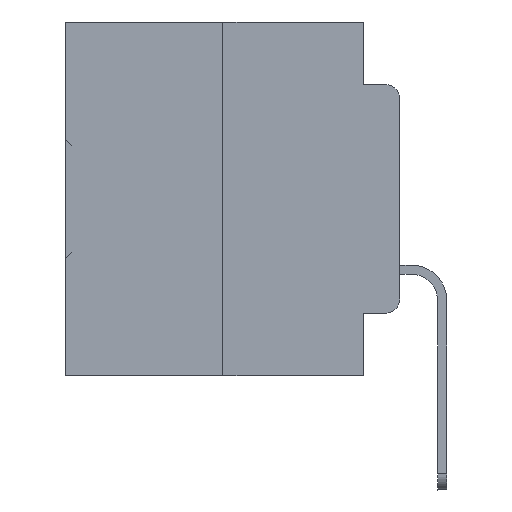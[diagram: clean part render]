
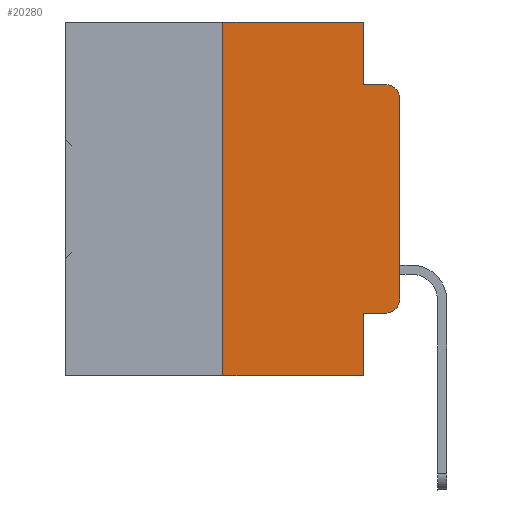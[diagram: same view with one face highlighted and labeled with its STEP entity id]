
A CAD part, left-side view. The second image highlights one B-rep face of the part: STEP entity #20280.
In plain terms, the highlighted planar face has unit normal (-1, 0, 0).
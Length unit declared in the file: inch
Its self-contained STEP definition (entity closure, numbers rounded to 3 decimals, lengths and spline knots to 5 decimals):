
#618 = AXIS2_PLACEMENT_3D ( 'NONE', #20040, #6520, #17661 ) ;
#851 = CARTESIAN_POINT ( 'NONE',  ( 0., 0.02, -0.4115 ) ) ;
#1379 = DIRECTION ( 'NONE',  ( 0., 0., -1. ) ) ;
#1526 = CARTESIAN_POINT ( 'NONE',  ( 0., 0.25, 0. ) ) ;
#1710 = CARTESIAN_POINT ( 'NONE',  ( 0., 0.051, -0.0885 ) ) ;
#2265 = ORIENTED_EDGE ( 'NONE', *, *, #16473, .T. ) ;
#2361 = CARTESIAN_POINT ( 'NONE',  ( 0., 0.051, -0.4115 ) ) ;
#2882 = CARTESIAN_POINT ( 'NONE',  ( 0., 0., -0.1085 ) ) ;
#3224 = CARTESIAN_POINT ( 'NONE',  ( 0., 0., 0. ) ) ;
#3629 = DIRECTION ( 'NONE',  ( 0., -1., 0. ) ) ;
#3813 = EDGE_CURVE ( 'NONE', #18099, #14512, #25123, .T. ) ;
#4417 = CIRCLE ( 'NONE', #24845, 0.02 ) ;
#4718 = ORIENTED_EDGE ( 'NONE', *, *, #17599, .F. ) ;
#5018 = LINE ( 'NONE', #29694, #18980 ) ;
#5337 = CARTESIAN_POINT ( 'NONE',  ( 0., 0.051, -0.0885 ) ) ;
#5689 = ORIENTED_EDGE ( 'NONE', *, *, #7912, .T. ) ;
#6039 = EDGE_CURVE ( 'NONE', #20537, #18242, #18977, .T. ) ;
#6078 = CARTESIAN_POINT ( 'NONE',  ( 0., 0.473, 0. ) ) ;
#6345 = VERTEX_POINT ( 'NONE', #35201 ) ;
#6520 = DIRECTION ( 'NONE',  ( -1., 0., 0. ) ) ;
#7912 = EDGE_CURVE ( 'NONE', #11514, #18099, #28253, .T. ) ;
#7952 = VERTEX_POINT ( 'NONE', #26760 ) ;
#8638 = ORIENTED_EDGE ( 'NONE', *, *, #23252, .F. ) ;
#9908 = LINE ( 'NONE', #1526, #12635 ) ;
#10779 = VECTOR ( 'NONE', #3629, 39.37008 ) ;
#11375 = VECTOR ( 'NONE', #15768, 39.37008 ) ;
#11440 = VECTOR ( 'NONE', #13870, 39.37008 ) ;
#11514 = VERTEX_POINT ( 'NONE', #32963 ) ;
#12531 = CARTESIAN_POINT ( 'NONE',  ( 0., 0.051, 0. ) ) ;
#12635 = VECTOR ( 'NONE', #18687, 39.37008 ) ;
#12728 = CARTESIAN_POINT ( 'NONE',  ( 0., 0.02, -0.0885 ) ) ;
#13870 = DIRECTION ( 'NONE',  ( 0., -1., 0. ) ) ;
#14045 = LINE ( 'NONE', #16439, #11440 ) ;
#14361 = DIRECTION ( 'NONE',  ( 0., 0., 1. ) ) ;
#14377 = EDGE_CURVE ( 'NONE', #32153, #6345, #20064, .T. ) ;
#14512 = VERTEX_POINT ( 'NONE', #12728 ) ;
#14769 = CARTESIAN_POINT ( 'NONE',  ( 0., 0.473, 0. ) ) ;
#15307 = AXIS2_PLACEMENT_3D ( 'NONE', #6078, #30933, #22912 ) ;
#15614 = EDGE_CURVE ( 'NONE', #23180, #7952, #14045, .T. ) ;
#15768 = DIRECTION ( 'NONE',  ( 0., -1., 0. ) ) ;
#16319 = EDGE_CURVE ( 'NONE', #20537, #7952, #5018, .T. ) ;
#16439 = CARTESIAN_POINT ( 'NONE',  ( 0., 0.473, -0.5 ) ) ;
#16473 = EDGE_CURVE ( 'NONE', #18242, #11514, #4417, .T. ) ;
#17599 = EDGE_CURVE ( 'NONE', #23180, #32153, #9908, .T. ) ;
#17661 = DIRECTION ( 'NONE',  ( 0., 0., -1. ) ) ;
#17719 = VERTEX_POINT ( 'NONE', #5337 ) ;
#18099 = VERTEX_POINT ( 'NONE', #2882 ) ;
#18242 = VERTEX_POINT ( 'NONE', #851 ) ;
#18687 = DIRECTION ( 'NONE',  ( 0., 0., 1. ) ) ;
#18718 = VECTOR ( 'NONE', #30494, 39.37008 ) ;
#18977 = LINE ( 'NONE', #2361, #18718 ) ;
#18980 = VECTOR ( 'NONE', #1379, 39.37008 ) ;
#19744 = ORIENTED_EDGE ( 'NONE', *, *, #15614, .T. ) ;
#20040 = CARTESIAN_POINT ( 'NONE',  ( 0., 0.02, -0.1085 ) ) ;
#20064 = LINE ( 'NONE', #14769, #10779 ) ;
#20280 = ADVANCED_FACE ( 'NONE', ( #33663 ), #33301, .F. ) ;
#20537 = VERTEX_POINT ( 'NONE', #30174 ) ;
#21416 = EDGE_CURVE ( 'NONE', #6345, #17719, #24251, .T. ) ;
#22382 = CARTESIAN_POINT ( 'NONE',  ( 0., 0.02, -0.3915 ) ) ;
#22390 = EDGE_LOOP ( 'NONE', ( #5689, #30524, #8638, #25232, #30759, #4718, #19744, #27698, #31379, #2265 ) ) ;
#22912 = DIRECTION ( 'NONE',  ( 0., 0., -1. ) ) ;
#23180 = VERTEX_POINT ( 'NONE', #32055 ) ;
#23252 = EDGE_CURVE ( 'NONE', #17719, #14512, #30209, .T. ) ;
#24251 = LINE ( 'NONE', #12531, #35205 ) ;
#24366 = VECTOR ( 'NONE', #14361, 39.37008 ) ;
#24845 = AXIS2_PLACEMENT_3D ( 'NONE', #22382, #33686, #33500 ) ;
#25123 = CIRCLE ( 'NONE', #618, 0.02 ) ;
#25232 = ORIENTED_EDGE ( 'NONE', *, *, #21416, .F. ) ;
#26760 = CARTESIAN_POINT ( 'NONE',  ( 0., 0.051, -0.5 ) ) ;
#27698 = ORIENTED_EDGE ( 'NONE', *, *, #16319, .F. ) ;
#28253 = LINE ( 'NONE', #3224, #24366 ) ;
#29694 = CARTESIAN_POINT ( 'NONE',  ( 0., 0.051, 0. ) ) ;
#30174 = CARTESIAN_POINT ( 'NONE',  ( 0., 0.051, -0.4115 ) ) ;
#30209 = LINE ( 'NONE', #1710, #11375 ) ;
#30494 = DIRECTION ( 'NONE',  ( 0., -1., 0. ) ) ;
#30524 = ORIENTED_EDGE ( 'NONE', *, *, #3813, .T. ) ;
#30759 = ORIENTED_EDGE ( 'NONE', *, *, #14377, .F. ) ;
#30933 = DIRECTION ( 'NONE',  ( 1., 0., 0. ) ) ;
#31159 = CARTESIAN_POINT ( 'NONE',  ( 0., 0.25, 0. ) ) ;
#31379 = ORIENTED_EDGE ( 'NONE', *, *, #6039, .T. ) ;
#32055 = CARTESIAN_POINT ( 'NONE',  ( 0., 0.25, -0.5 ) ) ;
#32153 = VERTEX_POINT ( 'NONE', #31159 ) ;
#32963 = CARTESIAN_POINT ( 'NONE',  ( 0., 0., -0.3915 ) ) ;
#33301 = PLANE ( 'NONE',  #15307 ) ;
#33500 = DIRECTION ( 'NONE',  ( 0., 0., -1. ) ) ;
#33663 = FACE_OUTER_BOUND ( 'NONE', #22390, .T. ) ;
#33686 = DIRECTION ( 'NONE',  ( -1., 0., 0. ) ) ;
#35201 = CARTESIAN_POINT ( 'NONE',  ( 0., 0.051, 0. ) ) ;
#35205 = VECTOR ( 'NONE', #35375, 39.37008 ) ;
#35375 = DIRECTION ( 'NONE',  ( 0., 0., -1. ) ) ;
